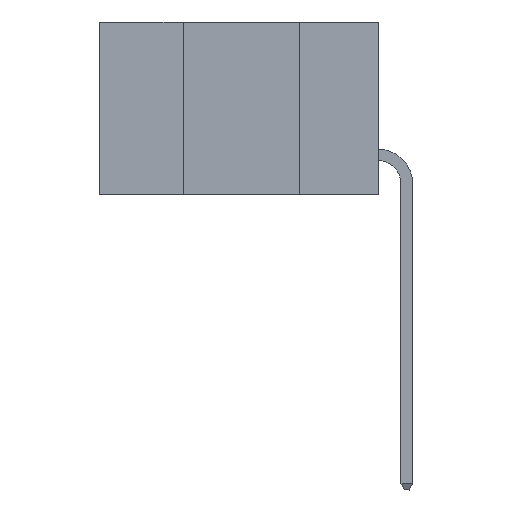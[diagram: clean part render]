
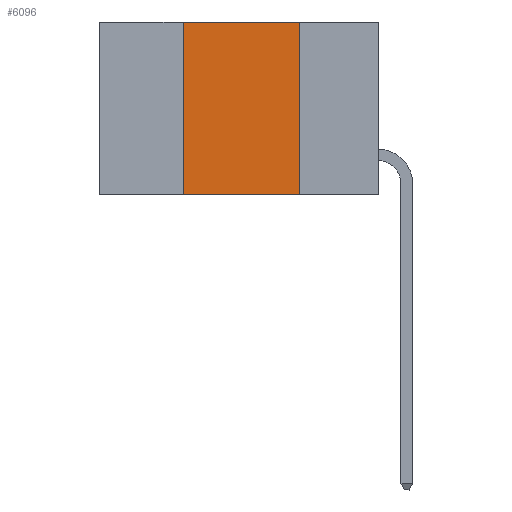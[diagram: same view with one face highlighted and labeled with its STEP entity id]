
A CAD part, left-side view. The second image highlights one B-rep face of the part: STEP entity #6096.
In plain terms, the highlighted planar face has unit normal (-1, 0, 0).
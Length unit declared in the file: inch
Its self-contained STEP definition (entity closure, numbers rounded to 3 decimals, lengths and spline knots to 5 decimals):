
#129 = EDGE_CURVE ( 'NONE', #6105, #399, #7892, .T. ) ;
#399 = VERTEX_POINT ( 'NONE', #1257 ) ;
#536 = LINE ( 'NONE', #8312, #13390 ) ;
#685 = ORIENTED_EDGE ( 'NONE', *, *, #129, .F. ) ;
#999 = CARTESIAN_POINT ( 'NONE',  ( 0., 0.42, 0. ) ) ;
#1257 = CARTESIAN_POINT ( 'NONE',  ( 0., 0.17, 0. ) ) ;
#3101 = ORIENTED_EDGE ( 'NONE', *, *, #4710, .F. ) ;
#3474 = DIRECTION ( 'NONE',  ( 1., 0., 0. ) ) ;
#3856 = EDGE_CURVE ( 'NONE', #399, #4996, #536, .T. ) ;
#3913 = ORIENTED_EDGE ( 'NONE', *, *, #3856, .F. ) ;
#4055 = FACE_OUTER_BOUND ( 'NONE', #4716, .T. ) ;
#4522 = LINE ( 'NONE', #999, #13360 ) ;
#4646 = VECTOR ( 'NONE', #12166, 39.37008 ) ;
#4710 = EDGE_CURVE ( 'NONE', #10027, #6105, #4522, .T. ) ;
#4716 = EDGE_LOOP ( 'NONE', ( #3913, #685, #3101, #11687 ) ) ;
#4888 = LINE ( 'NONE', #14374, #5645 ) ;
#4996 = VERTEX_POINT ( 'NONE', #15006 ) ;
#5524 = EDGE_CURVE ( 'NONE', #10027, #4996, #4888, .T. ) ;
#5645 = VECTOR ( 'NONE', #10488, 39.37008 ) ;
#5940 = CARTESIAN_POINT ( 'NONE',  ( 0., 0.6, 0. ) ) ;
#5997 = CARTESIAN_POINT ( 'NONE',  ( 0., 0.42, 0. ) ) ;
#6096 = ADVANCED_FACE ( 'NONE', ( #4055 ), #10787, .F. ) ;
#6105 = VERTEX_POINT ( 'NONE', #5997 ) ;
#7892 = LINE ( 'NONE', #11896, #4646 ) ;
#8043 = DIRECTION ( 'NONE',  ( 0., 0., 1. ) ) ;
#8312 = CARTESIAN_POINT ( 'NONE',  ( 0., 0.17, 0. ) ) ;
#10027 = VERTEX_POINT ( 'NONE', #14389 ) ;
#10488 = DIRECTION ( 'NONE',  ( 0., -1., 0. ) ) ;
#10524 = DIRECTION ( 'NONE',  ( 0., 0., -1. ) ) ;
#10787 = PLANE ( 'NONE',  #13164 ) ;
#11687 = ORIENTED_EDGE ( 'NONE', *, *, #5524, .T. ) ;
#11896 = CARTESIAN_POINT ( 'NONE',  ( 0., 0.6, 0. ) ) ;
#11980 = DIRECTION ( 'NONE',  ( 0., 0., -1. ) ) ;
#12166 = DIRECTION ( 'NONE',  ( 0., -1., 0. ) ) ;
#13164 = AXIS2_PLACEMENT_3D ( 'NONE', #5940, #3474, #11980 ) ;
#13360 = VECTOR ( 'NONE', #8043, 39.37008 ) ;
#13390 = VECTOR ( 'NONE', #10524, 39.37008 ) ;
#14374 = CARTESIAN_POINT ( 'NONE',  ( 0., 0.6, -0.37 ) ) ;
#14389 = CARTESIAN_POINT ( 'NONE',  ( 0., 0.42, -0.37 ) ) ;
#15006 = CARTESIAN_POINT ( 'NONE',  ( 0., 0.17, -0.37 ) ) ;
